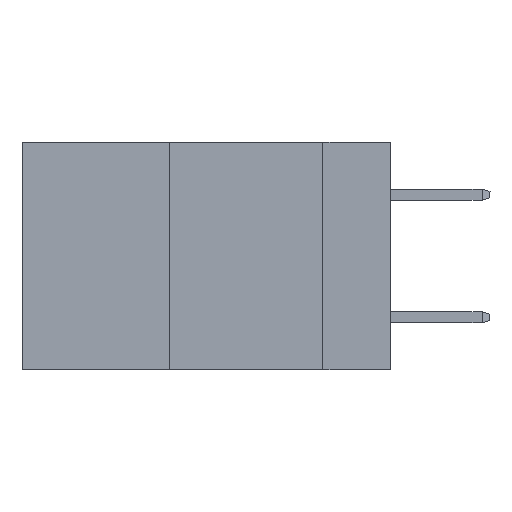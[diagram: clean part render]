
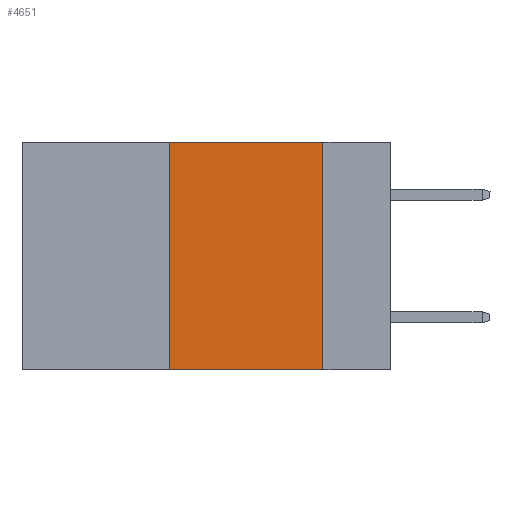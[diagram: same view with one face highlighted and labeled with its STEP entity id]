
A CAD part, left-side view. The second image highlights one B-rep face of the part: STEP entity #4651.
In plain terms, the highlighted planar face has unit normal (-1, 0, 0).
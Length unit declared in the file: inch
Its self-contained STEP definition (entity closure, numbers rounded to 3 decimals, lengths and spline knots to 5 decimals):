
#284 = CARTESIAN_POINT ( 'NONE',  ( 0., 0.11, -0.37 ) ) ;
#1091 = LINE ( 'NONE', #3728, #9207 ) ;
#1659 = LINE ( 'NONE', #9053, #6619 ) ;
#2865 = CARTESIAN_POINT ( 'NONE',  ( 0., 0.6, 0. ) ) ;
#3404 = CARTESIAN_POINT ( 'NONE',  ( 0., 0.6, -0.37 ) ) ;
#3681 = EDGE_CURVE ( 'NONE', #4567, #7733, #4415, .T. ) ;
#3728 = CARTESIAN_POINT ( 'NONE',  ( 0., 0.6, 0. ) ) ;
#3831 = DIRECTION ( 'NONE',  ( 0., 0., -1. ) ) ;
#3893 = VECTOR ( 'NONE', #8798, 39.37008 ) ;
#3956 = DIRECTION ( 'NONE',  ( 0., 0., -1. ) ) ;
#4406 = EDGE_CURVE ( 'NONE', #4567, #8049, #12181, .T. ) ;
#4415 = LINE ( 'NONE', #3404, #9659 ) ;
#4567 = VERTEX_POINT ( 'NONE', #4870 ) ;
#4651 = ADVANCED_FACE ( 'NONE', ( #6487 ), #8097, .F. ) ;
#4795 = DIRECTION ( 'NONE',  ( 0., -1., 0. ) ) ;
#4870 = CARTESIAN_POINT ( 'NONE',  ( 0., 0.36, -0.37 ) ) ;
#5583 = DIRECTION ( 'NONE',  ( 0., -1., 0. ) ) ;
#5792 = EDGE_CURVE ( 'NONE', #8272, #7733, #1659, .T. ) ;
#6066 = ORIENTED_EDGE ( 'NONE', *, *, #5792, .F. ) ;
#6118 = ORIENTED_EDGE ( 'NONE', *, *, #9770, .F. ) ;
#6134 = ORIENTED_EDGE ( 'NONE', *, *, #4406, .F. ) ;
#6166 = ORIENTED_EDGE ( 'NONE', *, *, #3681, .T. ) ;
#6487 = FACE_OUTER_BOUND ( 'NONE', #9684, .T. ) ;
#6619 = VECTOR ( 'NONE', #3831, 39.37008 ) ;
#7733 = VERTEX_POINT ( 'NONE', #284 ) ;
#7736 = CARTESIAN_POINT ( 'NONE',  ( 0., 0.36, 0. ) ) ;
#8049 = VERTEX_POINT ( 'NONE', #9168 ) ;
#8097 = PLANE ( 'NONE',  #11076 ) ;
#8272 = VERTEX_POINT ( 'NONE', #10798 ) ;
#8798 = DIRECTION ( 'NONE',  ( 0., 0., 1. ) ) ;
#9053 = CARTESIAN_POINT ( 'NONE',  ( 0., 0.11, 0. ) ) ;
#9168 = CARTESIAN_POINT ( 'NONE',  ( 0., 0.36, 0. ) ) ;
#9207 = VECTOR ( 'NONE', #4795, 39.37008 ) ;
#9659 = VECTOR ( 'NONE', #5583, 39.37008 ) ;
#9684 = EDGE_LOOP ( 'NONE', ( #6066, #6118, #6134, #6166 ) ) ;
#9770 = EDGE_CURVE ( 'NONE', #8049, #8272, #1091, .T. ) ;
#10226 = DIRECTION ( 'NONE',  ( 1., 0., 0. ) ) ;
#10798 = CARTESIAN_POINT ( 'NONE',  ( 0., 0.11, 0. ) ) ;
#11076 = AXIS2_PLACEMENT_3D ( 'NONE', #2865, #10226, #3956 ) ;
#12181 = LINE ( 'NONE', #7736, #3893 ) ;
